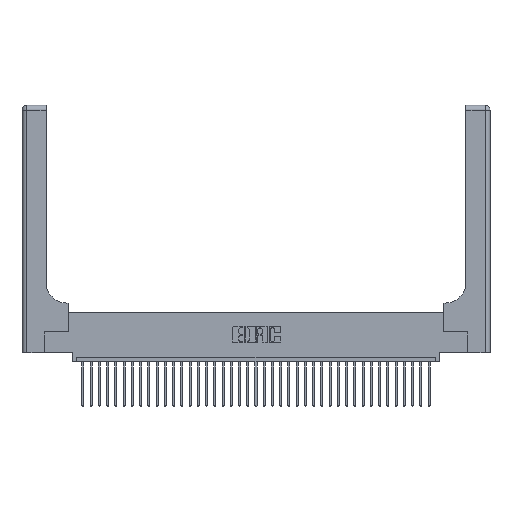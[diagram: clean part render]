
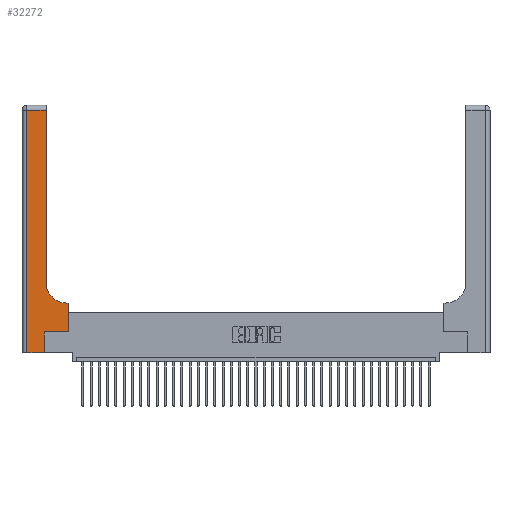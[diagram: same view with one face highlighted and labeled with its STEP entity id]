
A CAD part, top view. The second image highlights one B-rep face of the part: STEP entity #32272.
In plain terms, the highlighted planar face has unit normal (0, 0, 1).
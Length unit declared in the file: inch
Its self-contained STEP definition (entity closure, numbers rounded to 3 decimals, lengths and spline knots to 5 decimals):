
#30 = CARTESIAN_POINT ( 'NONE',  ( 0.269, 0.25, 0.37 ) ) ;
#182 = VECTOR ( 'NONE', #26987, 39.37008 ) ;
#556 = CARTESIAN_POINT ( 'NONE',  ( 0.5415, 0.6, 0.37 ) ) ;
#1138 = LINE ( 'NONE', #21000, #182 ) ;
#1486 = ORIENTED_EDGE ( 'NONE', *, *, #28489, .T. ) ;
#2356 = DIRECTION ( 'NONE',  ( 0., 0., -1. ) ) ;
#2400 = ORIENTED_EDGE ( 'NONE', *, *, #8254, .T. ) ;
#3019 = VERTEX_POINT ( 'NONE', #16587 ) ;
#3562 = EDGE_CURVE ( 'NONE', #20979, #17159, #32155, .T. ) ;
#3784 = EDGE_CURVE ( 'NONE', #7776, #16281, #8190, .T. ) ;
#4072 = CARTESIAN_POINT ( 'NONE',  ( 0.06, 2.94, 0.37 ) ) ;
#5077 = ORIENTED_EDGE ( 'NONE', *, *, #18844, .T. ) ;
#5978 = EDGE_CURVE ( 'NONE', #27957, #3019, #1138, .T. ) ;
#6372 = FACE_OUTER_BOUND ( 'NONE', #6752, .T. ) ;
#6545 = DIRECTION ( 'NONE',  ( 0., 1., 0. ) ) ;
#6752 = EDGE_LOOP ( 'NONE', ( #8951, #32278, #9466, #5077, #26371, #23076, #1486, #20949, #2400 ) ) ;
#6826 = LINE ( 'NONE', #15125, #22203 ) ;
#7178 = DIRECTION ( 'NONE',  ( 0., 0., -1. ) ) ;
#7776 = VERTEX_POINT ( 'NONE', #21843 ) ;
#7944 = DIRECTION ( 'NONE',  ( 1., 0., 0. ) ) ;
#8074 = CARTESIAN_POINT ( 'NONE',  ( 0.5415, 0.85, 0.37 ) ) ;
#8190 = LINE ( 'NONE', #30263, #14924 ) ;
#8254 = EDGE_CURVE ( 'NONE', #16281, #27957, #14075, .T. ) ;
#8951 = ORIENTED_EDGE ( 'NONE', *, *, #5978, .T. ) ;
#9466 = ORIENTED_EDGE ( 'NONE', *, *, #3562, .T. ) ;
#9777 = VECTOR ( 'NONE', #18178, 39.37008 ) ;
#10764 = LINE ( 'NONE', #30, #17504 ) ;
#12319 = EDGE_CURVE ( 'NONE', #29651, #17298, #30633, .T. ) ;
#12507 = DIRECTION ( 'NONE',  ( -1., 0., 0. ) ) ;
#12598 = CARTESIAN_POINT ( 'NONE',  ( 0., 3., 0.37 ) ) ;
#14075 = CIRCLE ( 'NONE', #20077, 0.25 ) ;
#14251 = CARTESIAN_POINT ( 'NONE',  ( 0.269, 0., 0.37 ) ) ;
#14924 = VECTOR ( 'NONE', #18997, 39.37008 ) ;
#15125 = CARTESIAN_POINT ( 'NONE',  ( 0.5585, 0.25, 0.37 ) ) ;
#15866 = DIRECTION ( 'NONE',  ( -1., 0., 0. ) ) ;
#16281 = VERTEX_POINT ( 'NONE', #556 ) ;
#16587 = CARTESIAN_POINT ( 'NONE',  ( 0.2915, 2.94, 0.37 ) ) ;
#17159 = VERTEX_POINT ( 'NONE', #22004 ) ;
#17298 = VERTEX_POINT ( 'NONE', #31018 ) ;
#17504 = VECTOR ( 'NONE', #20013, 39.37008 ) ;
#17569 = EDGE_CURVE ( 'NONE', #3019, #20979, #20539, .T. ) ;
#18178 = DIRECTION ( 'NONE',  ( 0., 1., 0. ) ) ;
#18844 = EDGE_CURVE ( 'NONE', #17159, #29651, #25828, .T. ) ;
#18926 = AXIS2_PLACEMENT_3D ( 'NONE', #12598, #7178, #15866 ) ;
#18997 = DIRECTION ( 'NONE',  ( -1., 0., 0. ) ) ;
#20013 = DIRECTION ( 'NONE',  ( 1., 0., 0. ) ) ;
#20077 = AXIS2_PLACEMENT_3D ( 'NONE', #8074, #2356, #7944 ) ;
#20539 = LINE ( 'NONE', #35872, #25039 ) ;
#20949 = ORIENTED_EDGE ( 'NONE', *, *, #3784, .T. ) ;
#20979 = VERTEX_POINT ( 'NONE', #4072 ) ;
#21000 = CARTESIAN_POINT ( 'NONE',  ( 0.2915, 3., 0.37 ) ) ;
#21843 = CARTESIAN_POINT ( 'NONE',  ( 0.5585, 0.6, 0.37 ) ) ;
#22004 = CARTESIAN_POINT ( 'NONE',  ( 0.06, 0., 0.37 ) ) ;
#22203 = VECTOR ( 'NONE', #6545, 39.37008 ) ;
#22624 = DIRECTION ( 'NONE',  ( 1., 0., 0. ) ) ;
#23076 = ORIENTED_EDGE ( 'NONE', *, *, #24003, .T. ) ;
#24003 = EDGE_CURVE ( 'NONE', #17298, #34489, #10764, .T. ) ;
#24520 = CARTESIAN_POINT ( 'NONE',  ( 0.269, 0., 0.37 ) ) ;
#25039 = VECTOR ( 'NONE', #12507, 39.37008 ) ;
#25828 = LINE ( 'NONE', #28545, #27664 ) ;
#26371 = ORIENTED_EDGE ( 'NONE', *, *, #12319, .T. ) ;
#26987 = DIRECTION ( 'NONE',  ( 0., 1., 0. ) ) ;
#27664 = VECTOR ( 'NONE', #22624, 39.37008 ) ;
#27957 = VERTEX_POINT ( 'NONE', #28913 ) ;
#28147 = CARTESIAN_POINT ( 'NONE',  ( 0.06, 3., 0.37 ) ) ;
#28489 = EDGE_CURVE ( 'NONE', #34489, #7776, #6826, .T. ) ;
#28545 = CARTESIAN_POINT ( 'NONE',  ( 0., 0., 0.37 ) ) ;
#28913 = CARTESIAN_POINT ( 'NONE',  ( 0.2915, 0.85, 0.37 ) ) ;
#29651 = VERTEX_POINT ( 'NONE', #24520 ) ;
#30263 = CARTESIAN_POINT ( 'NONE',  ( 0.2915, 0.6, 0.37 ) ) ;
#30351 = VECTOR ( 'NONE', #36181, 39.37008 ) ;
#30633 = LINE ( 'NONE', #14251, #9777 ) ;
#31018 = CARTESIAN_POINT ( 'NONE',  ( 0.269, 0.25, 0.37 ) ) ;
#31603 = CARTESIAN_POINT ( 'NONE',  ( 0.5585, 0.25, 0.37 ) ) ;
#32155 = LINE ( 'NONE', #28147, #30351 ) ;
#32272 = ADVANCED_FACE ( 'NONE', ( #6372 ), #36092, .F. ) ;
#32278 = ORIENTED_EDGE ( 'NONE', *, *, #17569, .T. ) ;
#34489 = VERTEX_POINT ( 'NONE', #31603 ) ;
#35872 = CARTESIAN_POINT ( 'NONE',  ( 0., 2.94, 0.37 ) ) ;
#36092 = PLANE ( 'NONE',  #18926 ) ;
#36181 = DIRECTION ( 'NONE',  ( 0., -1., 0. ) ) ;
